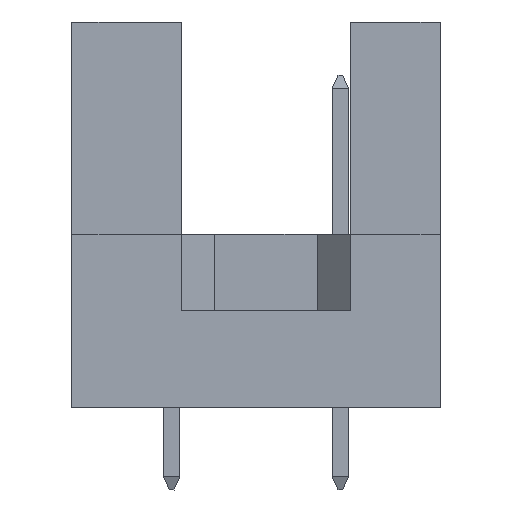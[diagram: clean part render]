
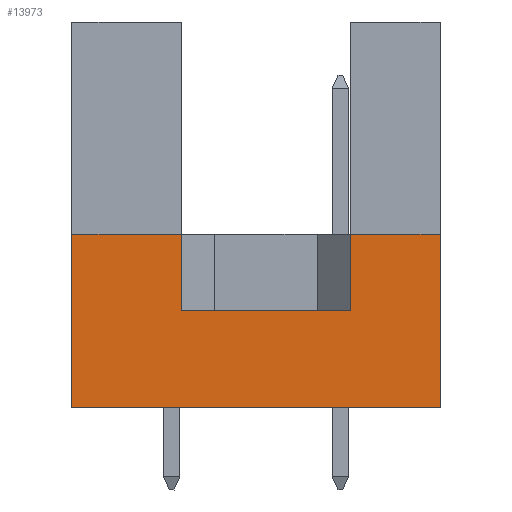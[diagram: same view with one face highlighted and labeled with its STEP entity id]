
A CAD part, left-side view. The second image highlights one B-rep face of the part: STEP entity #13973.
In plain terms, the highlighted planar face has unit normal (-1, 0, 0).
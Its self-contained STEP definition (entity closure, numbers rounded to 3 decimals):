
#281 = LINE ( 'NONE', #4083, #1708 ) ;
#467 = DIRECTION ( 'NONE',  ( 0., -1., 0. ) ) ;
#471 = CARTESIAN_POINT ( 'NONE',  ( -47.5, 2.71, 5.2 ) ) ;
#702 = VECTOR ( 'NONE', #467, 1000. ) ;
#768 = VERTEX_POINT ( 'NONE', #471 ) ;
#980 = VECTOR ( 'NONE', #8368, 1000. ) ;
#1008 = EDGE_CURVE ( 'NONE', #4336, #3818, #9731, .T. ) ;
#1036 = PLANE ( 'NONE',  #9679 ) ;
#1397 = ORIENTED_EDGE ( 'NONE', *, *, #10008, .F. ) ;
#1552 = CARTESIAN_POINT ( 'NONE',  ( -47.5, 0., 0. ) ) ;
#1708 = VECTOR ( 'NONE', #5158, 1000. ) ;
#1901 = VERTEX_POINT ( 'NONE', #14608 ) ;
#1951 = ORIENTED_EDGE ( 'NONE', *, *, #12823, .F. ) ;
#1974 = VECTOR ( 'NONE', #7602, 1000. ) ;
#2041 = LINE ( 'NONE', #3361, #702 ) ;
#2121 = CARTESIAN_POINT ( 'NONE',  ( -47.5, 11.1, 5.2 ) ) ;
#2275 = CARTESIAN_POINT ( 'NONE',  ( -47.5, 0., 0. ) ) ;
#2553 = LINE ( 'NONE', #5009, #1974 ) ;
#3361 = CARTESIAN_POINT ( 'NONE',  ( -47.5, 7.79, 2.9 ) ) ;
#3482 = DIRECTION ( 'NONE',  ( 0., -1., 0. ) ) ;
#3607 = DIRECTION ( 'NONE',  ( 0., 0., -1. ) ) ;
#3818 = VERTEX_POINT ( 'NONE', #14845 ) ;
#4083 = CARTESIAN_POINT ( 'NONE',  ( -47.5, 11.1, 0. ) ) ;
#4216 = ORIENTED_EDGE ( 'NONE', *, *, #14832, .T. ) ;
#4251 = VECTOR ( 'NONE', #10569, 1000. ) ;
#4336 = VERTEX_POINT ( 'NONE', #5882 ) ;
#4441 = VERTEX_POINT ( 'NONE', #8939 ) ;
#4709 = ORIENTED_EDGE ( 'NONE', *, *, #14173, .F. ) ;
#5009 = CARTESIAN_POINT ( 'NONE',  ( -47.5, 2.71, 2.9 ) ) ;
#5158 = DIRECTION ( 'NONE',  ( 0., 0., 1. ) ) ;
#5185 = EDGE_CURVE ( 'NONE', #16298, #4441, #8998, .T. ) ;
#5522 = ORIENTED_EDGE ( 'NONE', *, *, #13755, .F. ) ;
#5564 = ORIENTED_EDGE ( 'NONE', *, *, #13459, .T. ) ;
#5882 = CARTESIAN_POINT ( 'NONE',  ( -47.5, 11.1, 5.2 ) ) ;
#6016 = LINE ( 'NONE', #12564, #6503 ) ;
#6116 = LINE ( 'NONE', #8614, #13399 ) ;
#6463 = VERTEX_POINT ( 'NONE', #8920 ) ;
#6503 = VECTOR ( 'NONE', #13725, 1000. ) ;
#6935 = CARTESIAN_POINT ( 'NONE',  ( -47.5, 7.79, 2.9 ) ) ;
#7602 = DIRECTION ( 'NONE',  ( 0., 0., 1. ) ) ;
#7859 = ORIENTED_EDGE ( 'NONE', *, *, #1008, .F. ) ;
#8368 = DIRECTION ( 'NONE',  ( 0., -1., 0. ) ) ;
#8614 = CARTESIAN_POINT ( 'NONE',  ( -47.5, 11.1, 5.2 ) ) ;
#8920 = CARTESIAN_POINT ( 'NONE',  ( -47.5, 2.71, 2.9 ) ) ;
#8939 = CARTESIAN_POINT ( 'NONE',  ( -47.5, 0., 5.2 ) ) ;
#8998 = LINE ( 'NONE', #1552, #4251 ) ;
#9303 = EDGE_LOOP ( 'NONE', ( #5522, #5564, #7859, #1951, #4216, #14765, #4709, #1397 ) ) ;
#9602 = CARTESIAN_POINT ( 'NONE',  ( -47.5, 11.1, 0. ) ) ;
#9679 = AXIS2_PLACEMENT_3D ( 'NONE', #16359, #16039, #3607 ) ;
#9729 = FACE_OUTER_BOUND ( 'NONE', #9303, .T. ) ;
#9731 = LINE ( 'NONE', #2121, #13048 ) ;
#10008 = EDGE_CURVE ( 'NONE', #6463, #768, #2553, .T. ) ;
#10336 = VERTEX_POINT ( 'NONE', #6935 ) ;
#10569 = DIRECTION ( 'NONE',  ( 0., 0., 1. ) ) ;
#12180 = LINE ( 'NONE', #9602, #980 ) ;
#12564 = CARTESIAN_POINT ( 'NONE',  ( -47.5, 7.79, 2.9 ) ) ;
#12823 = EDGE_CURVE ( 'NONE', #1901, #4336, #281, .T. ) ;
#13048 = VECTOR ( 'NONE', #14535, 1000. ) ;
#13399 = VECTOR ( 'NONE', #3482, 1000. ) ;
#13459 = EDGE_CURVE ( 'NONE', #10336, #3818, #6016, .T. ) ;
#13725 = DIRECTION ( 'NONE',  ( 0., 0., 1. ) ) ;
#13755 = EDGE_CURVE ( 'NONE', #10336, #6463, #2041, .T. ) ;
#13973 = ADVANCED_FACE ( 'NONE', ( #9729 ), #1036, .F. ) ;
#14173 = EDGE_CURVE ( 'NONE', #768, #4441, #6116, .T. ) ;
#14535 = DIRECTION ( 'NONE',  ( 0., -1., 0. ) ) ;
#14608 = CARTESIAN_POINT ( 'NONE',  ( -47.5, 11.1, 0. ) ) ;
#14765 = ORIENTED_EDGE ( 'NONE', *, *, #5185, .T. ) ;
#14832 = EDGE_CURVE ( 'NONE', #1901, #16298, #12180, .T. ) ;
#14845 = CARTESIAN_POINT ( 'NONE',  ( -47.5, 7.79, 5.2 ) ) ;
#16039 = DIRECTION ( 'NONE',  ( 1., 0., 0. ) ) ;
#16298 = VERTEX_POINT ( 'NONE', #2275 ) ;
#16359 = CARTESIAN_POINT ( 'NONE',  ( -47.5, 11.1, 0. ) ) ;
